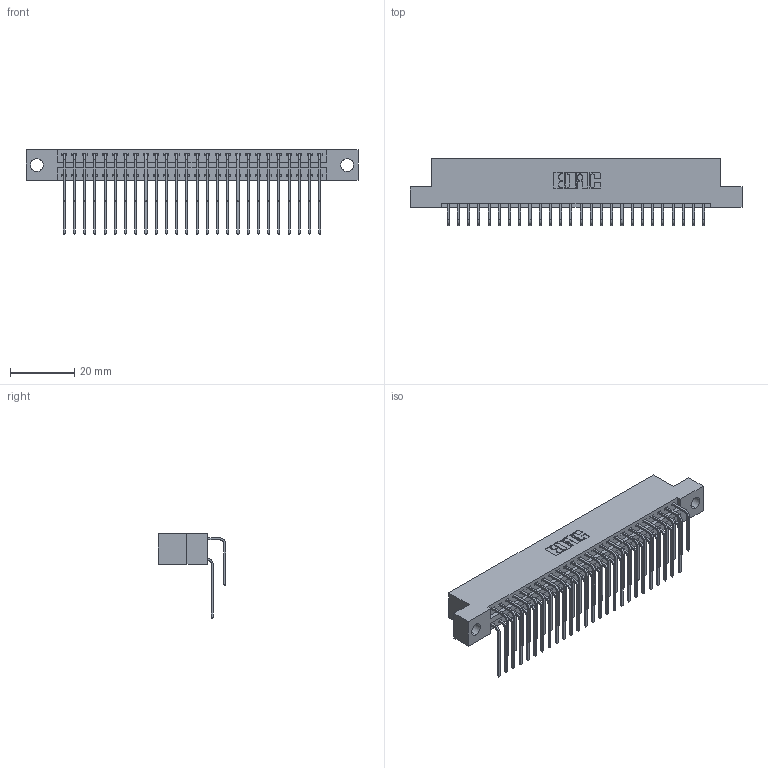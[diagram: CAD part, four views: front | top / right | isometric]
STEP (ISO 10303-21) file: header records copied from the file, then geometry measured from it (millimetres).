
FILE_DESCRIPTION (( 'STEP AP203' ), '1' );
FILE_NAME ('396-052-559-204.STEP', '2019-11-03T08:51:46', ( '' ), ( '' ), 'SwSTEP 2.0', 'SolidWorks 2016', '' );
FILE_SCHEMA (( 'CONFIG_CONTROL_DESIGN' ));
Length unit declared in the file: inch
Products named in the file (4): 345-292-001_558 559 Tail - 1; 396-052-559-204; 345-292-001_559 Tail - 2; 346 Part_Flush Mounting Lugs - 0.156 Dia-TH
Assembly tree (53 placements, depth 2):
  396-052-559-204
    346 Part_Flush Mounting Lugs - 0.156 Dia-TH
    345-292-001_558 559 Tail - 1  x26
    345-292-001_559 Tail - 2  x26
Bounding box: 103.12 x 20.89 x 26.16 mm (x, y, z)
Volume: 10143.7 mm3; surface area: 14944.2 mm2
Topology: 53 solids, 53 shells, 2930 faces, 8701 edges, 5730 vertices
Faces by surface type: plane 2000, cylinder 930
Entity records: 20909 total; most frequent: CARTESIAN_POINT 3519, ORIENTED_EDGE 3402, DIRECTION 3125, EDGE_CURVE 1701, VECTOR 1425, LINE 1425, VERTEX_POINT 1130, AXIS2_PLACEMENT_3D 850
